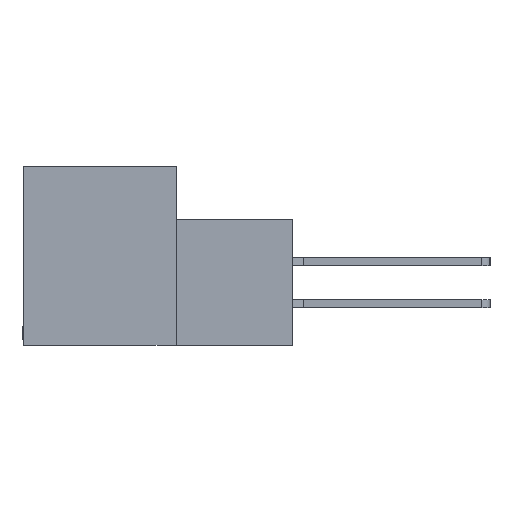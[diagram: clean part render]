
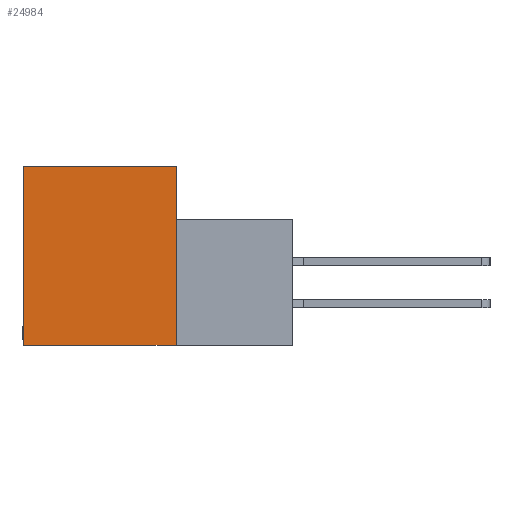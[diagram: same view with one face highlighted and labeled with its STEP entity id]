
A CAD part, left-side view. The second image highlights one B-rep face of the part: STEP entity #24984.
In plain terms, the highlighted planar face has unit normal (-1, 0, 0).
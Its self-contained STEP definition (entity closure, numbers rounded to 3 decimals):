
#1261 = DIRECTION ( 'NONE',  ( 0., 0., 1. ) ) ;
#1763 = LINE ( 'NONE', #33747, #29477 ) ;
#4614 = DIRECTION ( 'NONE',  ( 1., 0., 0. ) ) ;
#5356 = EDGE_CURVE ( 'NONE', #26382, #13442, #25480, .T. ) ;
#6150 = CARTESIAN_POINT ( 'NONE',  ( 0., 0., 0. ) ) ;
#7889 = CARTESIAN_POINT ( 'NONE',  ( 0., 0., 0. ) ) ;
#9662 = DIRECTION ( 'NONE',  ( 0., 0., -1. ) ) ;
#9801 = EDGE_CURVE ( 'NONE', #13442, #31602, #29983, .T. ) ;
#10902 = VECTOR ( 'NONE', #18483, 1000. ) ;
#11070 = DIRECTION ( 'NONE',  ( 0., 1., 0. ) ) ;
#11303 = ORIENTED_EDGE ( 'NONE', *, *, #5356, .F. ) ;
#12126 = EDGE_CURVE ( 'NONE', #21470, #26382, #18049, .T. ) ;
#13195 = CARTESIAN_POINT ( 'NONE',  ( 0., 11.506, 0. ) ) ;
#13442 = VERTEX_POINT ( 'NONE', #31891 ) ;
#14010 = FACE_OUTER_BOUND ( 'NONE', #26600, .T. ) ;
#15070 = PLANE ( 'NONE',  #31858 ) ;
#16842 = CARTESIAN_POINT ( 'NONE',  ( 0., -8.814, -13.487 ) ) ;
#18049 = LINE ( 'NONE', #31884, #10902 ) ;
#18483 = DIRECTION ( 'NONE',  ( 0., -1., 0. ) ) ;
#19581 = ORIENTED_EDGE ( 'NONE', *, *, #12126, .F. ) ;
#21470 = VERTEX_POINT ( 'NONE', #13195 ) ;
#24940 = ORIENTED_EDGE ( 'NONE', *, *, #9801, .F. ) ;
#24984 = ADVANCED_FACE ( 'NONE', ( #14010 ), #15070, .F. ) ;
#25480 = LINE ( 'NONE', #6150, #33444 ) ;
#26382 = VERTEX_POINT ( 'NONE', #7889 ) ;
#26600 = EDGE_LOOP ( 'NONE', ( #24940, #11303, #19581, #29029 ) ) ;
#28941 = CARTESIAN_POINT ( 'NONE',  ( 0., 0., 0. ) ) ;
#29029 = ORIENTED_EDGE ( 'NONE', *, *, #33309, .F. ) ;
#29477 = VECTOR ( 'NONE', #1261, 1000. ) ;
#29983 = LINE ( 'NONE', #16842, #31658 ) ;
#30583 = DIRECTION ( 'NONE',  ( 0., 0., -1. ) ) ;
#31602 = VERTEX_POINT ( 'NONE', #33635 ) ;
#31658 = VECTOR ( 'NONE', #11070, 1000. ) ;
#31858 = AXIS2_PLACEMENT_3D ( 'NONE', #28941, #4614, #9662 ) ;
#31884 = CARTESIAN_POINT ( 'NONE',  ( 0., 11.506, 0. ) ) ;
#31891 = CARTESIAN_POINT ( 'NONE',  ( 0., 0., -13.487 ) ) ;
#33309 = EDGE_CURVE ( 'NONE', #31602, #21470, #1763, .T. ) ;
#33444 = VECTOR ( 'NONE', #30583, 1000. ) ;
#33635 = CARTESIAN_POINT ( 'NONE',  ( 0., 11.506, -13.487 ) ) ;
#33747 = CARTESIAN_POINT ( 'NONE',  ( 0., 11.506, -13.487 ) ) ;
